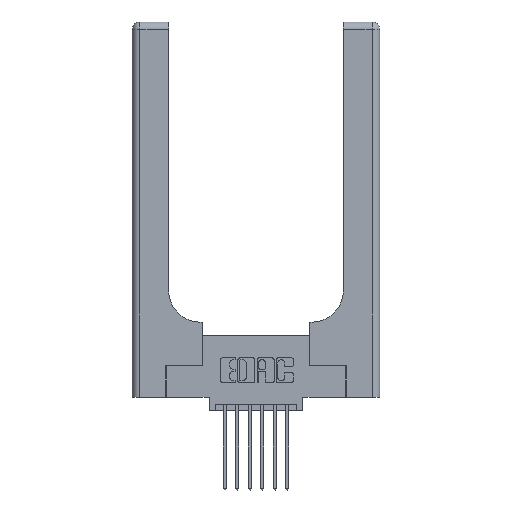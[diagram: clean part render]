
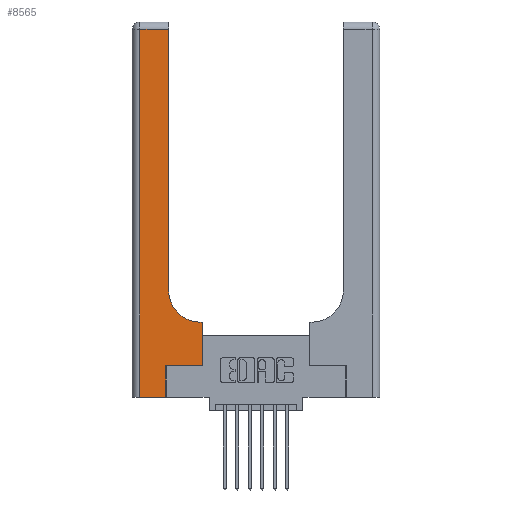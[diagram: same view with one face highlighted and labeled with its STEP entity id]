
A CAD part, top view. The second image highlights one B-rep face of the part: STEP entity #8565.
In plain terms, the highlighted planar face has unit normal (0, 0, 1).
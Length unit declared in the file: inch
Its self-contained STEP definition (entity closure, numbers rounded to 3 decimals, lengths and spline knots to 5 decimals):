
#257 = EDGE_CURVE ( 'NONE', #8912, #10938, #7909, .T. ) ;
#365 = CARTESIAN_POINT ( 'NONE',  ( 0.5585, 0.6, 0.37 ) ) ;
#366 = ORIENTED_EDGE ( 'NONE', *, *, #8018, .T. ) ;
#1396 = LINE ( 'NONE', #1535, #13295 ) ;
#1515 = CARTESIAN_POINT ( 'NONE',  ( 0.06, 0., 0.37 ) ) ;
#1535 = CARTESIAN_POINT ( 'NONE',  ( 0.269, 0., 0.37 ) ) ;
#1536 = LINE ( 'NONE', #8182, #10388 ) ;
#1670 = PLANE ( 'NONE',  #12772 ) ;
#1741 = LINE ( 'NONE', #13141, #7513 ) ;
#1754 = DIRECTION ( 'NONE',  ( 1., 0., 0. ) ) ;
#1812 = EDGE_CURVE ( 'NONE', #6861, #12762, #11146, .T. ) ;
#1849 = LINE ( 'NONE', #1884, #7617 ) ;
#1884 = CARTESIAN_POINT ( 'NONE',  ( 0.2915, 0.6, 0.37 ) ) ;
#2051 = CARTESIAN_POINT ( 'NONE',  ( 0.269, 0., 0.37 ) ) ;
#2096 = EDGE_CURVE ( 'NONE', #12762, #6305, #1396, .T. ) ;
#2355 = ORIENTED_EDGE ( 'NONE', *, *, #3352, .T. ) ;
#2544 = DIRECTION ( 'NONE',  ( 0., 1., 0. ) ) ;
#2574 = EDGE_CURVE ( 'NONE', #10701, #6861, #1741, .T. ) ;
#2928 = CARTESIAN_POINT ( 'NONE',  ( 0., 0., 0.37 ) ) ;
#3352 = EDGE_CURVE ( 'NONE', #9072, #10701, #1536, .T. ) ;
#3441 = DIRECTION ( 'NONE',  ( 0., 1., 0. ) ) ;
#3442 = ORIENTED_EDGE ( 'NONE', *, *, #3455, .T. ) ;
#3455 = EDGE_CURVE ( 'NONE', #14116, #11075, #6252, .T. ) ;
#4064 = DIRECTION ( 'NONE',  ( 0., 0., -1. ) ) ;
#4782 = DIRECTION ( 'NONE',  ( -1., 0., 0. ) ) ;
#4937 = DIRECTION ( 'NONE',  ( 1., 0., 0. ) ) ;
#5442 = ORIENTED_EDGE ( 'NONE', *, *, #2574, .T. ) ;
#5817 = ORIENTED_EDGE ( 'NONE', *, *, #1812, .T. ) ;
#6163 = ORIENTED_EDGE ( 'NONE', *, *, #2096, .T. ) ;
#6252 = LINE ( 'NONE', #7168, #11992 ) ;
#6305 = VERTEX_POINT ( 'NONE', #8444 ) ;
#6333 = CARTESIAN_POINT ( 'NONE',  ( 0., 3., 0.37 ) ) ;
#6515 = ORIENTED_EDGE ( 'NONE', *, *, #13308, .T. ) ;
#6859 = LINE ( 'NONE', #7228, #12609 ) ;
#6861 = VERTEX_POINT ( 'NONE', #1515 ) ;
#6865 = ORIENTED_EDGE ( 'NONE', *, *, #257, .T. ) ;
#7154 = CARTESIAN_POINT ( 'NONE',  ( 0.06, 2.94, 0.37 ) ) ;
#7168 = CARTESIAN_POINT ( 'NONE',  ( 0.5585, 0.25, 0.37 ) ) ;
#7228 = CARTESIAN_POINT ( 'NONE',  ( 0.269, 0.25, 0.37 ) ) ;
#7511 = DIRECTION ( 'NONE',  ( 0., 1., 0. ) ) ;
#7513 = VECTOR ( 'NONE', #12918, 39.37008 ) ;
#7617 = VECTOR ( 'NONE', #8781, 39.37008 ) ;
#7909 = CIRCLE ( 'NONE', #11265, 0.25 ) ;
#8018 = EDGE_CURVE ( 'NONE', #6305, #14116, #6859, .T. ) ;
#8076 = VECTOR ( 'NONE', #1754, 39.37008 ) ;
#8182 = CARTESIAN_POINT ( 'NONE',  ( 0., 2.94, 0.37 ) ) ;
#8444 = CARTESIAN_POINT ( 'NONE',  ( 0.269, 0.25, 0.37 ) ) ;
#8565 = ADVANCED_FACE ( 'NONE', ( #9175 ), #1670, .F. ) ;
#8781 = DIRECTION ( 'NONE',  ( -1., 0., 0. ) ) ;
#8912 = VERTEX_POINT ( 'NONE', #10445 ) ;
#9072 = VERTEX_POINT ( 'NONE', #12988 ) ;
#9175 = FACE_OUTER_BOUND ( 'NONE', #13635, .T. ) ;
#9621 = VECTOR ( 'NONE', #7511, 39.37008 ) ;
#10388 = VECTOR ( 'NONE', #4782, 39.37008 ) ;
#10445 = CARTESIAN_POINT ( 'NONE',  ( 0.5415, 0.6, 0.37 ) ) ;
#10701 = VERTEX_POINT ( 'NONE', #7154 ) ;
#10938 = VERTEX_POINT ( 'NONE', #14547 ) ;
#10951 = CARTESIAN_POINT ( 'NONE',  ( 0.2915, 3., 0.37 ) ) ;
#11075 = VERTEX_POINT ( 'NONE', #365 ) ;
#11146 = LINE ( 'NONE', #2928, #8076 ) ;
#11265 = AXIS2_PLACEMENT_3D ( 'NONE', #13212, #13868, #13063 ) ;
#11768 = CARTESIAN_POINT ( 'NONE',  ( 0.5585, 0.25, 0.37 ) ) ;
#11992 = VECTOR ( 'NONE', #2544, 39.37008 ) ;
#12100 = DIRECTION ( 'NONE',  ( -1., 0., 0. ) ) ;
#12609 = VECTOR ( 'NONE', #4937, 39.37008 ) ;
#12670 = LINE ( 'NONE', #10951, #9621 ) ;
#12762 = VERTEX_POINT ( 'NONE', #2051 ) ;
#12772 = AXIS2_PLACEMENT_3D ( 'NONE', #6333, #4064, #12100 ) ;
#12918 = DIRECTION ( 'NONE',  ( 0., -1., 0. ) ) ;
#12988 = CARTESIAN_POINT ( 'NONE',  ( 0.2915, 2.94, 0.37 ) ) ;
#13063 = DIRECTION ( 'NONE',  ( 1., 0., 0. ) ) ;
#13141 = CARTESIAN_POINT ( 'NONE',  ( 0.06, 3., 0.37 ) ) ;
#13212 = CARTESIAN_POINT ( 'NONE',  ( 0.5415, 0.85, 0.37 ) ) ;
#13295 = VECTOR ( 'NONE', #3441, 39.37008 ) ;
#13308 = EDGE_CURVE ( 'NONE', #11075, #8912, #1849, .T. ) ;
#13635 = EDGE_LOOP ( 'NONE', ( #14227, #2355, #5442, #5817, #6163, #366, #3442, #6515, #6865 ) ) ;
#13868 = DIRECTION ( 'NONE',  ( 0., 0., -1. ) ) ;
#14116 = VERTEX_POINT ( 'NONE', #11768 ) ;
#14227 = ORIENTED_EDGE ( 'NONE', *, *, #14824, .T. ) ;
#14547 = CARTESIAN_POINT ( 'NONE',  ( 0.2915, 0.85, 0.37 ) ) ;
#14824 = EDGE_CURVE ( 'NONE', #10938, #9072, #12670, .T. ) ;
